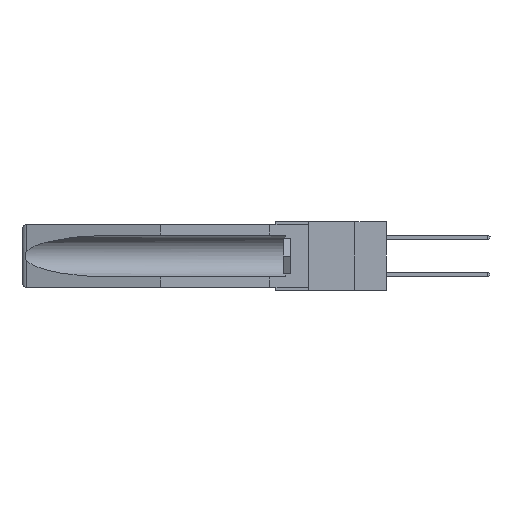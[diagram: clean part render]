
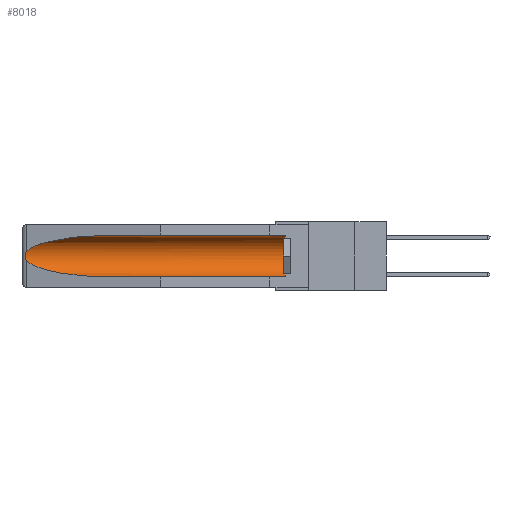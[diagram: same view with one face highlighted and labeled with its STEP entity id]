
A CAD part, left-side view. The second image highlights one B-rep face of the part: STEP entity #8018.
In plain terms, the highlighted cylindrical face has radius 2.857 mm (diameter 5.715 mm), a partial arc.
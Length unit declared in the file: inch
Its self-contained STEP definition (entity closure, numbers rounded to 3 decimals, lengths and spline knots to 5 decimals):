
#197 = LINE ( 'NONE', #6577, #14119 ) ;
#312 = VERTEX_POINT ( 'NONE', #22167 ) ;
#362 = CARTESIAN_POINT ( 'NONE',  ( 0.155, -0.30754, -0.059 ) ) ;
#813 = ORIENTED_EDGE ( 'NONE', *, *, #14514, .T. ) ;
#937 =( BOUNDED_CURVE ( )  B_SPLINE_CURVE ( 3, ( #22791, #18663, #24838, #12740 ),
 .UNSPECIFIED., .F., .T. ) 
 B_SPLINE_CURVE_WITH_KNOTS ( ( 4, 4 ),
 ( 4.71239, 6.08839 ),
 .UNSPECIFIED. ) 
 CURVE ( )  GEOMETRIC_REPRESENTATION_ITEM ( )  RATIONAL_B_SPLINE_CURVE ( ( 1., 0.848, 0.848, 1. ) ) 
 REPRESENTATION_ITEM ( '' )  );
#1515 = CARTESIAN_POINT ( 'NONE',  ( 0.26537, 1.52718, -0.19328 ) ) ;
#1686 = CARTESIAN_POINT ( 'NONE',  ( 0.2675, 1.53308, -0.17534 ) ) ;
#1771 = CARTESIAN_POINT ( 'NONE',  ( 0.26597, 1.52961, -0.15275 ) ) ;
#1859 = CARTESIAN_POINT ( 'NONE',  ( 0.26655, 1.53094, -0.18657 ) ) ;
#2368 = EDGE_CURVE ( 'NONE', #25318, #312, #937, .T. ) ;
#2481 = CIRCLE ( 'NONE', #8440, 0.1125 ) ;
#3239 = ORIENTED_EDGE ( 'NONE', *, *, #25760, .T. ) ;
#3559 = CARTESIAN_POINT ( 'NONE',  ( 0.26537, 1.52718, -0.14972 ) ) ;
#4746 = CARTESIAN_POINT ( 'NONE',  ( 0.21114, 1.30732, -0.284 ) ) ;
#6577 = CARTESIAN_POINT ( 'NONE',  ( 0.155, -0.30754, -0.284 ) ) ;
#8018 = ADVANCED_FACE ( 'NONE', ( #8377 ), #14757, .F. ) ;
#8377 = FACE_OUTER_BOUND ( 'NONE', #12526, .T. ) ;
#8419 = DIRECTION ( 'NONE',  ( 0., 1., 0. ) ) ;
#8440 = AXIS2_PLACEMENT_3D ( 'NONE', #16874, #16779, #14572 ) ;
#8749 = CARTESIAN_POINT ( 'NONE',  ( 0.25451, 1.48313, -0.24835 ) ) ;
#10297 = ORIENTED_EDGE ( 'NONE', *, *, #17652, .F. ) ;
#11465 = CARTESIAN_POINT ( 'NONE',  ( 0.155, 0.126, -0.284 ) ) ;
#11931 = VERTEX_POINT ( 'NONE', #17104 ) ;
#12279 = DIRECTION ( 'NONE',  ( 0., 0., 1. ) ) ;
#12526 = EDGE_LOOP ( 'NONE', ( #18083, #3239, #18082, #10297, #24858, #813 ) ) ;
#12740 = CARTESIAN_POINT ( 'NONE',  ( 0.26537, 1.52718, -0.14972 ) ) ;
#12790 = CARTESIAN_POINT ( 'NONE',  ( 0.155, 0.126, -0.059 ) ) ;
#13736 = AXIS2_PLACEMENT_3D ( 'NONE', #20294, #24240, #12279 ) ;
#13742 = LINE ( 'NONE', #362, #20701 ) ;
#13983 = CARTESIAN_POINT ( 'NONE',  ( 0.26654, 1.53092, -0.15636 ) ) ;
#14047 =( BOUNDED_CURVE ( )  B_SPLINE_CURVE ( 3, ( #14780, #8749, #4746, #16796 ),
 .UNSPECIFIED., .F., .F. ) 
 B_SPLINE_CURVE_WITH_KNOTS ( ( 4, 4 ),
 ( 0.1948, 1.5708 ),
 .UNSPECIFIED. ) 
 CURVE ( )  GEOMETRIC_REPRESENTATION_ITEM ( )  RATIONAL_B_SPLINE_CURVE ( ( 1., 0.848, 0.848, 1. ) ) 
 REPRESENTATION_ITEM ( '' )  );
#14119 = VECTOR ( 'NONE', #14928, 39.37008 ) ;
#14514 = EDGE_CURVE ( 'NONE', #18339, #25318, #13742, .T. ) ;
#14572 = DIRECTION ( 'NONE',  ( 0., 0., 1. ) ) ;
#14757 = CYLINDRICAL_SURFACE ( 'NONE', #13736, 0.1125 ) ;
#14780 = CARTESIAN_POINT ( 'NONE',  ( 0.26537, 1.52718, -0.19328 ) ) ;
#14928 = DIRECTION ( 'NONE',  ( 0., 1., 0. ) ) ;
#16161 = EDGE_CURVE ( 'NONE', #25679, #18339, #2481, .T. ) ;
#16779 = DIRECTION ( 'NONE',  ( 0., -1., 0. ) ) ;
#16796 = CARTESIAN_POINT ( 'NONE',  ( 0.155, 1.07973, -0.284 ) ) ;
#16874 = CARTESIAN_POINT ( 'NONE',  ( 0.155, 0.126, -0.1715 ) ) ;
#17104 = CARTESIAN_POINT ( 'NONE',  ( 0.155, 1.07973, -0.284 ) ) ;
#17652 = EDGE_CURVE ( 'NONE', #25679, #11931, #197, .T. ) ;
#18082 = ORIENTED_EDGE ( 'NONE', *, *, #26022, .T. ) ;
#18083 = ORIENTED_EDGE ( 'NONE', *, *, #2368, .T. ) ;
#18339 = VERTEX_POINT ( 'NONE', #12790 ) ;
#18663 = CARTESIAN_POINT ( 'NONE',  ( 0.21114, 1.30732, -0.059 ) ) ;
#19885 = CARTESIAN_POINT ( 'NONE',  ( 0.2673, 1.5327, -0.16383 ) ) ;
#20278 = CARTESIAN_POINT ( 'NONE',  ( 0.155, 1.07973, -0.059 ) ) ;
#20294 = CARTESIAN_POINT ( 'NONE',  ( 0.155, -0.30754, -0.1715 ) ) ;
#20701 = VECTOR ( 'NONE', #8419, 39.37008 ) ;
#21671 = CARTESIAN_POINT ( 'NONE',  ( 0.2675, 1.53308, -0.16763 ) ) ;
#22167 = CARTESIAN_POINT ( 'NONE',  ( 0.26537, 1.52718, -0.14972 ) ) ;
#22791 = CARTESIAN_POINT ( 'NONE',  ( 0.155, 1.07973, -0.059 ) ) ;
#23596 = VERTEX_POINT ( 'NONE', #24398 ) ;
#23666 = CARTESIAN_POINT ( 'NONE',  ( 0.26597, 1.5296, -0.19026 ) ) ;
#23876 = B_SPLINE_CURVE_WITH_KNOTS ( 'NONE', 3,
 ( #3559, #1771, #13983, #19885, #21671, #1686, #23929, #1859, #23666, #1515 ),
 .UNSPECIFIED., .F., .F.,
 ( 4, 2, 2, 2, 4 ),
 ( 0., 0.00029, 0.00058, 0.00087, 0.00117 ),
 .UNSPECIFIED. ) ;
#23929 = CARTESIAN_POINT ( 'NONE',  ( 0.2673, 1.53269, -0.17917 ) ) ;
#24240 = DIRECTION ( 'NONE',  ( 0., 1., 0. ) ) ;
#24398 = CARTESIAN_POINT ( 'NONE',  ( 0.26537, 1.52718, -0.19328 ) ) ;
#24838 = CARTESIAN_POINT ( 'NONE',  ( 0.25451, 1.48313, -0.09465 ) ) ;
#24858 = ORIENTED_EDGE ( 'NONE', *, *, #16161, .T. ) ;
#25318 = VERTEX_POINT ( 'NONE', #20278 ) ;
#25679 = VERTEX_POINT ( 'NONE', #11465 ) ;
#25760 = EDGE_CURVE ( 'NONE', #312, #23596, #23876, .T. ) ;
#26022 = EDGE_CURVE ( 'NONE', #23596, #11931, #14047, .T. ) ;
